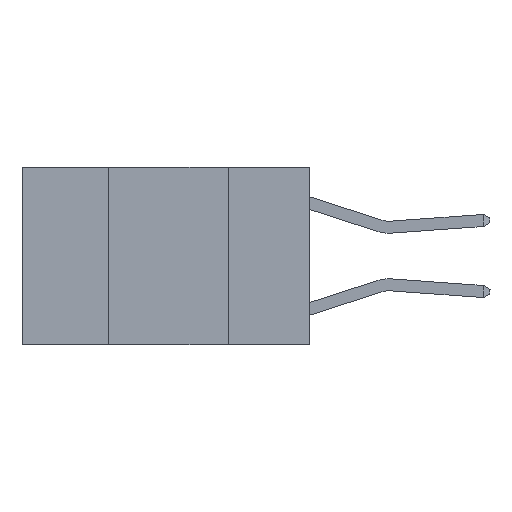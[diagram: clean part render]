
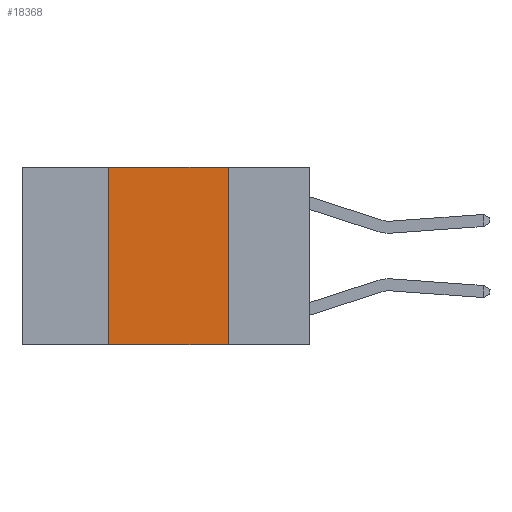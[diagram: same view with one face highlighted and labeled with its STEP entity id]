
A CAD part, left-side view. The second image highlights one B-rep face of the part: STEP entity #18368.
In plain terms, the highlighted planar face has unit normal (-1, 0, 0).
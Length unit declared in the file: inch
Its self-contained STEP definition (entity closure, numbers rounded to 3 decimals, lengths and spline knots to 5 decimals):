
#63 = DIRECTION ( 'NONE',  ( 1., 0., 0. ) ) ;
#863 = LINE ( 'NONE', #16392, #13439 ) ;
#1141 = ORIENTED_EDGE ( 'NONE', *, *, #12447, .F. ) ;
#2444 = ORIENTED_EDGE ( 'NONE', *, *, #16758, .F. ) ;
#3096 = VERTEX_POINT ( 'NONE', #10479 ) ;
#4066 = ORIENTED_EDGE ( 'NONE', *, *, #5309, .T. ) ;
#4276 = DIRECTION ( 'NONE',  ( 0., -1., 0. ) ) ;
#4705 = LINE ( 'NONE', #16824, #12713 ) ;
#5309 = EDGE_CURVE ( 'NONE', #6001, #16740, #863, .T. ) ;
#6001 = VERTEX_POINT ( 'NONE', #15812 ) ;
#7139 = DIRECTION ( 'NONE',  ( 0., -1., 0. ) ) ;
#9403 = CARTESIAN_POINT ( 'NONE',  ( 0., 0.6, 0. ) ) ;
#9621 = CARTESIAN_POINT ( 'NONE',  ( 0., 0.6, 0. ) ) ;
#10360 = VERTEX_POINT ( 'NONE', #15848 ) ;
#10479 = CARTESIAN_POINT ( 'NONE',  ( 0., 0.42, 0. ) ) ;
#10500 = VECTOR ( 'NONE', #15055, 39.37008 ) ;
#11183 = FACE_OUTER_BOUND ( 'NONE', #14789, .T. ) ;
#12295 = LINE ( 'NONE', #9403, #18567 ) ;
#12447 = EDGE_CURVE ( 'NONE', #6001, #3096, #4705, .T. ) ;
#12525 = DIRECTION ( 'NONE',  ( 0., 0., 1. ) ) ;
#12713 = VECTOR ( 'NONE', #12525, 39.37008 ) ;
#13403 = LINE ( 'NONE', #16869, #10500 ) ;
#13439 = VECTOR ( 'NONE', #7139, 39.37008 ) ;
#14307 = EDGE_CURVE ( 'NONE', #10360, #16740, #13403, .T. ) ;
#14789 = EDGE_LOOP ( 'NONE', ( #16686, #2444, #1141, #4066 ) ) ;
#15055 = DIRECTION ( 'NONE',  ( 0., 0., -1. ) ) ;
#15800 = PLANE ( 'NONE',  #16019 ) ;
#15812 = CARTESIAN_POINT ( 'NONE',  ( 0., 0.42, -0.37 ) ) ;
#15848 = CARTESIAN_POINT ( 'NONE',  ( 0., 0.17, 0. ) ) ;
#16019 = AXIS2_PLACEMENT_3D ( 'NONE', #9621, #63, #18657 ) ;
#16119 = CARTESIAN_POINT ( 'NONE',  ( 0., 0.17, -0.37 ) ) ;
#16392 = CARTESIAN_POINT ( 'NONE',  ( 0., 0.6, -0.37 ) ) ;
#16686 = ORIENTED_EDGE ( 'NONE', *, *, #14307, .F. ) ;
#16740 = VERTEX_POINT ( 'NONE', #16119 ) ;
#16758 = EDGE_CURVE ( 'NONE', #3096, #10360, #12295, .T. ) ;
#16824 = CARTESIAN_POINT ( 'NONE',  ( 0., 0.42, 0. ) ) ;
#16869 = CARTESIAN_POINT ( 'NONE',  ( 0., 0.17, 0. ) ) ;
#18368 = ADVANCED_FACE ( 'NONE', ( #11183 ), #15800, .F. ) ;
#18567 = VECTOR ( 'NONE', #4276, 39.37008 ) ;
#18657 = DIRECTION ( 'NONE',  ( 0., 0., -1. ) ) ;
